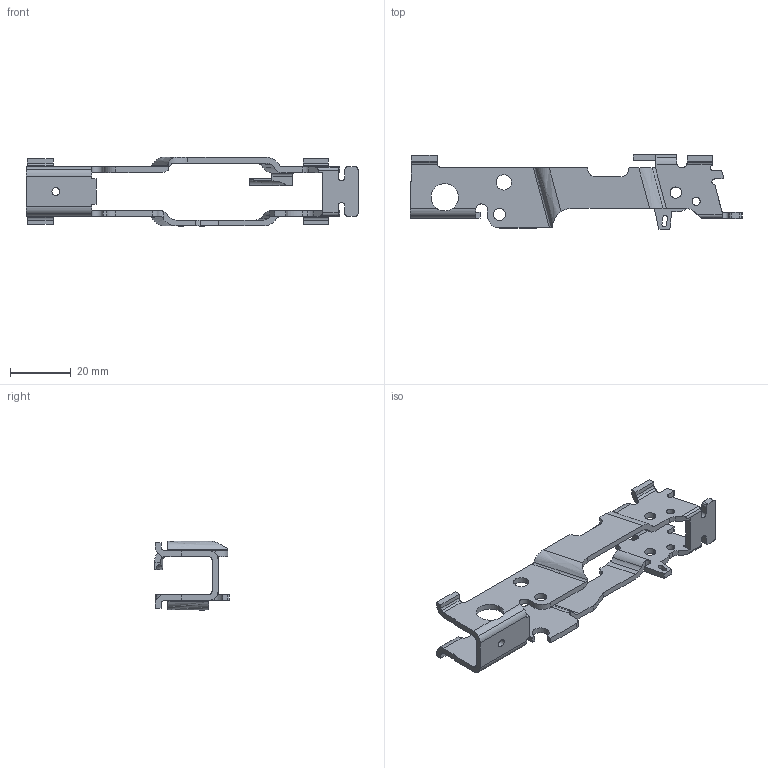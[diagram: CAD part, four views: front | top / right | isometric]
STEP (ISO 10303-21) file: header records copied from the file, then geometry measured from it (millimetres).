
FILE_DESCRIPTION (( 'STEP AP214' ), '1' );
FILE_NAME ('Frame.step', '2014-07-30T19:45:50', ( 'WarFairy' ), ( '' ), 'SwSTEP 2.0', 'SolidWorks 2013', '' );
FILE_SCHEMA (( 'AUTOMOTIVE_DESIGN' ));
Length unit declared in the file: millimetre
Products named in the file (1): Frame
Bounding box: 109.73 x 24.62 x 23.05 mm (x, y, z)
Volume: 6872.1 mm3; surface area: 8695 mm2
Topology: 1 solids, 1 shells, 240 faces, 715 edges, 473 vertices
Faces by surface type: cylinder 117, plane 106, torus 9, bspline 8
Entity records: 8354 total; most frequent: CARTESIAN_POINT 1788, ORIENTED_EDGE 1430, DIRECTION 1355, EDGE_CURVE 715, VERTEX_POINT 473, AXIS2_PLACEMENT_3D 472, LINE 411, VECTOR 411
